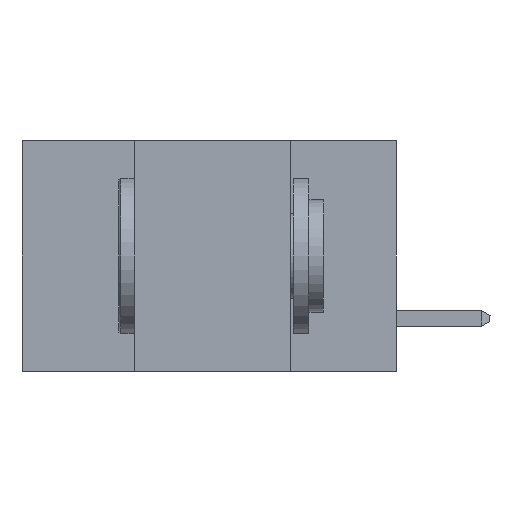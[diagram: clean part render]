
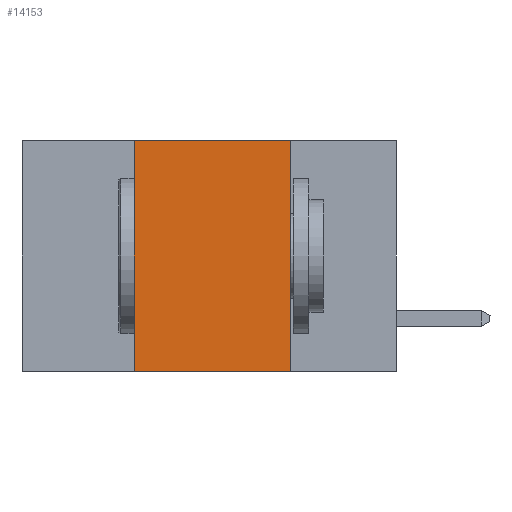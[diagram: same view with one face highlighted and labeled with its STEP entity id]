
A CAD part, left-side view. The second image highlights one B-rep face of the part: STEP entity #14153.
In plain terms, the highlighted planar face has unit normal (-1, 0, 0).
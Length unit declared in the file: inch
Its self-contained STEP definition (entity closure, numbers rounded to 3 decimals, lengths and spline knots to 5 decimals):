
#669 = ORIENTED_EDGE ( 'NONE', *, *, #9745, .T. ) ;
#1071 = EDGE_CURVE ( 'NONE', #3380, #16135, #17648, .T. ) ;
#1201 = CARTESIAN_POINT ( 'NONE',  ( 0., 0.6, 0. ) ) ;
#1530 = FACE_OUTER_BOUND ( 'NONE', #13497, .T. ) ;
#2088 = CARTESIAN_POINT ( 'NONE',  ( 0., 0.17, 0. ) ) ;
#2354 = VECTOR ( 'NONE', #13052, 39.37008 ) ;
#2715 = ORIENTED_EDGE ( 'NONE', *, *, #16670, .F. ) ;
#2829 = DIRECTION ( 'NONE',  ( 0., -1., 0. ) ) ;
#3380 = VERTEX_POINT ( 'NONE', #14680 ) ;
#4799 = CARTESIAN_POINT ( 'NONE',  ( 0., 0.42, -0.37 ) ) ;
#5239 = CARTESIAN_POINT ( 'NONE',  ( 0., 0.17, -0.37 ) ) ;
#5489 = CARTESIAN_POINT ( 'NONE',  ( 0., 0.17, -0.37 ) ) ;
#5492 = PLANE ( 'NONE',  #7174 ) ;
#6065 = LINE ( 'NONE', #5489, #10058 ) ;
#6458 = VERTEX_POINT ( 'NONE', #5239 ) ;
#6910 = DIRECTION ( 'NONE',  ( 0., 0., -1. ) ) ;
#6914 = DIRECTION ( 'NONE',  ( 0., 0., -1. ) ) ;
#7174 = AXIS2_PLACEMENT_3D ( 'NONE', #1201, #14914, #6914 ) ;
#8968 = CARTESIAN_POINT ( 'NONE',  ( 0., 0.42, -0.37 ) ) ;
#9745 = EDGE_CURVE ( 'NONE', #11914, #6458, #16634, .T. ) ;
#10058 = VECTOR ( 'NONE', #6910, 39.37008 ) ;
#11012 = VECTOR ( 'NONE', #16216, 39.37008 ) ;
#11662 = EDGE_CURVE ( 'NONE', #16135, #6458, #6065, .T. ) ;
#11914 = VERTEX_POINT ( 'NONE', #4799 ) ;
#13052 = DIRECTION ( 'NONE',  ( 0., 0., 1. ) ) ;
#13095 = VECTOR ( 'NONE', #2829, 39.37008 ) ;
#13256 = CARTESIAN_POINT ( 'NONE',  ( 0., 0.6, 0. ) ) ;
#13497 = EDGE_LOOP ( 'NONE', ( #16590, #16796, #2715, #669 ) ) ;
#14153 = ADVANCED_FACE ( 'NONE', ( #1530 ), #5492, .F. ) ;
#14680 = CARTESIAN_POINT ( 'NONE',  ( 0., 0.42, 0. ) ) ;
#14914 = DIRECTION ( 'NONE',  ( 1., 0., 0. ) ) ;
#15040 = CARTESIAN_POINT ( 'NONE',  ( 0., 0.6, -0.37 ) ) ;
#16135 = VERTEX_POINT ( 'NONE', #2088 ) ;
#16216 = DIRECTION ( 'NONE',  ( 0., -1., 0. ) ) ;
#16590 = ORIENTED_EDGE ( 'NONE', *, *, #11662, .F. ) ;
#16634 = LINE ( 'NONE', #15040, #13095 ) ;
#16670 = EDGE_CURVE ( 'NONE', #11914, #3380, #16827, .T. ) ;
#16796 = ORIENTED_EDGE ( 'NONE', *, *, #1071, .F. ) ;
#16827 = LINE ( 'NONE', #8968, #2354 ) ;
#17648 = LINE ( 'NONE', #13256, #11012 ) ;
